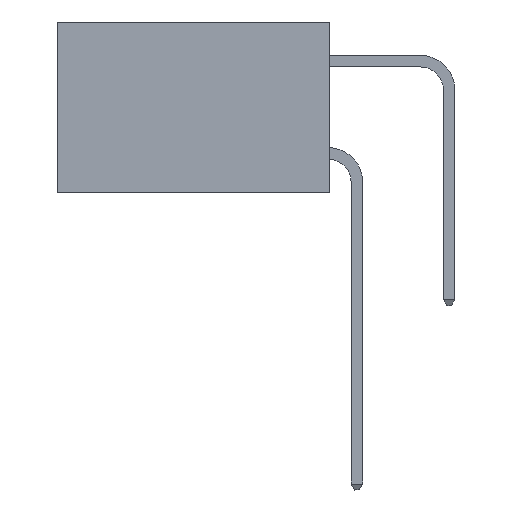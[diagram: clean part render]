
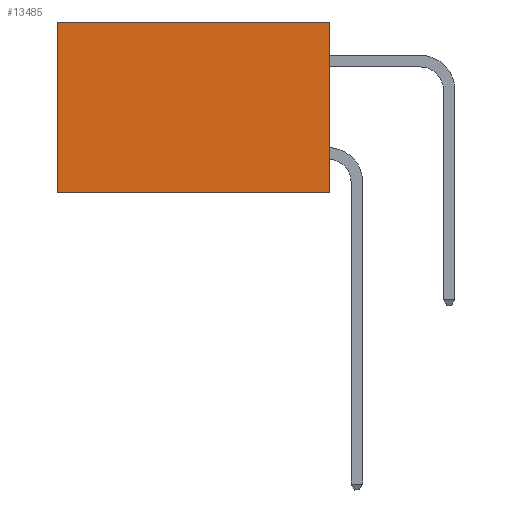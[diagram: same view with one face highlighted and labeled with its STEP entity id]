
A CAD part, left-side view. The second image highlights one B-rep face of the part: STEP entity #13485.
In plain terms, the highlighted planar face has unit normal (-1, 0, 0).
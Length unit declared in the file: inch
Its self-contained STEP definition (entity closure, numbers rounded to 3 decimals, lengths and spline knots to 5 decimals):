
#469 = VERTEX_POINT ( 'NONE', #15633 ) ;
#1431 = CARTESIAN_POINT ( 'NONE',  ( 0.277, 0., -0.37 ) ) ;
#1639 = CARTESIAN_POINT ( 'NONE',  ( 0.277, 0., -0.37 ) ) ;
#2902 = LINE ( 'NONE', #26643, #26015 ) ;
#3000 = ORIENTED_EDGE ( 'NONE', *, *, #20951, .F. ) ;
#3279 = DIRECTION ( 'NONE',  ( 1., 0., 0. ) ) ;
#5314 = FACE_OUTER_BOUND ( 'NONE', #13004, .T. ) ;
#6262 = LINE ( 'NONE', #1431, #10857 ) ;
#6324 = VECTOR ( 'NONE', #24654, 39.37008 ) ;
#8361 = DIRECTION ( 'NONE',  ( 0., 1., 0. ) ) ;
#10857 = VECTOR ( 'NONE', #14954, 39.37008 ) ;
#11727 = ORIENTED_EDGE ( 'NONE', *, *, #20086, .T. ) ;
#11984 = VERTEX_POINT ( 'NONE', #14200 ) ;
#12065 = LINE ( 'NONE', #1639, #23246 ) ;
#13004 = EDGE_LOOP ( 'NONE', ( #21166, #3000, #20016, #11727 ) ) ;
#13333 = DIRECTION ( 'NONE',  ( 0., 0., -1. ) ) ;
#13485 = ADVANCED_FACE ( 'NONE', ( #5314 ), #21155, .F. ) ;
#13899 = CARTESIAN_POINT ( 'NONE',  ( 0.277, 0.59, 0. ) ) ;
#14200 = CARTESIAN_POINT ( 'NONE',  ( 0.277, 0., 0. ) ) ;
#14954 = DIRECTION ( 'NONE',  ( 0., 0., -1. ) ) ;
#15633 = CARTESIAN_POINT ( 'NONE',  ( 0.277, 0.59, -0.37 ) ) ;
#16739 = CARTESIAN_POINT ( 'NONE',  ( 0.277, 0., -0.37 ) ) ;
#17683 = AXIS2_PLACEMENT_3D ( 'NONE', #16739, #3279, #18992 ) ;
#18992 = DIRECTION ( 'NONE',  ( 0., 0., -1. ) ) ;
#20016 = ORIENTED_EDGE ( 'NONE', *, *, #23014, .F. ) ;
#20086 = EDGE_CURVE ( 'NONE', #11984, #20621, #24212, .T. ) ;
#20426 = EDGE_CURVE ( 'NONE', #20621, #469, #2902, .T. ) ;
#20621 = VERTEX_POINT ( 'NONE', #13899 ) ;
#20951 = EDGE_CURVE ( 'NONE', #22517, #469, #12065, .T. ) ;
#21155 = PLANE ( 'NONE',  #17683 ) ;
#21166 = ORIENTED_EDGE ( 'NONE', *, *, #20426, .T. ) ;
#22470 = CARTESIAN_POINT ( 'NONE',  ( 0.277, 0., 0. ) ) ;
#22517 = VERTEX_POINT ( 'NONE', #26636 ) ;
#23014 = EDGE_CURVE ( 'NONE', #11984, #22517, #6262, .T. ) ;
#23246 = VECTOR ( 'NONE', #8361, 39.37008 ) ;
#24212 = LINE ( 'NONE', #22470, #6324 ) ;
#24654 = DIRECTION ( 'NONE',  ( 0., 1., 0. ) ) ;
#26015 = VECTOR ( 'NONE', #13333, 39.37008 ) ;
#26636 = CARTESIAN_POINT ( 'NONE',  ( 0.277, 0., -0.37 ) ) ;
#26643 = CARTESIAN_POINT ( 'NONE',  ( 0.277, 0.59, -0.37 ) ) ;
